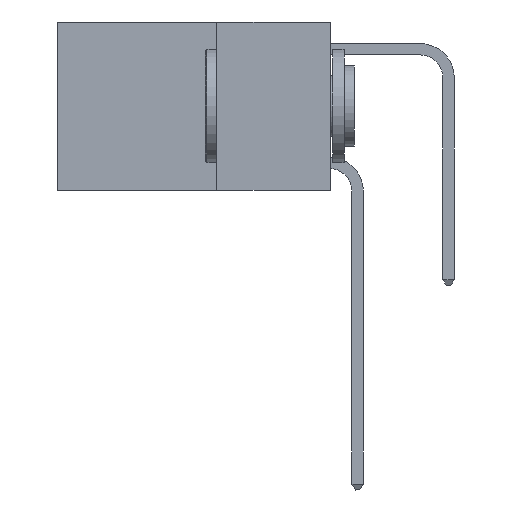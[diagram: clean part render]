
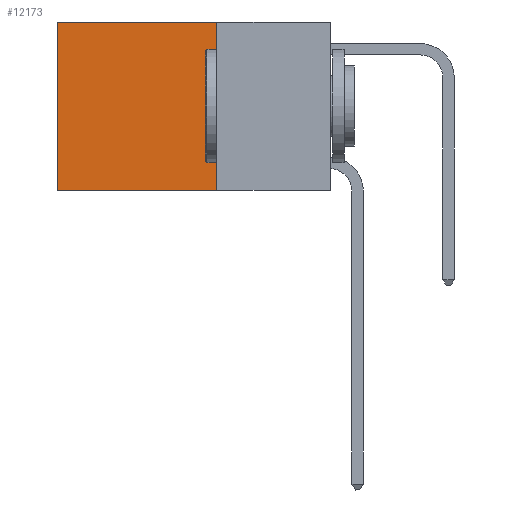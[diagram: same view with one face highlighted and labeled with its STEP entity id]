
A CAD part, left-side view. The second image highlights one B-rep face of the part: STEP entity #12173.
In plain terms, the highlighted planar face has unit normal (-1, 0, 0).
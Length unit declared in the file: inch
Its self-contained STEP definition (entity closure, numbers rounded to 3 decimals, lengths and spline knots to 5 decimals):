
#615 = VERTEX_POINT ( 'NONE', #9736 ) ;
#970 = EDGE_CURVE ( 'NONE', #3640, #1485, #16937, .T. ) ;
#1111 = DIRECTION ( 'NONE',  ( 0., 0., -1. ) ) ;
#1485 = VERTEX_POINT ( 'NONE', #8193 ) ;
#2724 = LINE ( 'NONE', #4094, #6900 ) ;
#2854 = DIRECTION ( 'NONE',  ( 0., 1., 0. ) ) ;
#3399 = EDGE_CURVE ( 'NONE', #615, #3640, #2724, .T. ) ;
#3640 = VERTEX_POINT ( 'NONE', #19001 ) ;
#4094 = CARTESIAN_POINT ( 'NONE',  ( 0.2625, 0.25, 0. ) ) ;
#4179 = CARTESIAN_POINT ( 'NONE',  ( 0.2625, 0.6, 0. ) ) ;
#4950 = AXIS2_PLACEMENT_3D ( 'NONE', #6698, #14297, #1111 ) ;
#5082 = ORIENTED_EDGE ( 'NONE', *, *, #23337, .T. ) ;
#5183 = ORIENTED_EDGE ( 'NONE', *, *, #970, .F. ) ;
#5208 = PLANE ( 'NONE',  #4950 ) ;
#5256 = CARTESIAN_POINT ( 'NONE',  ( 0.2625, 0.6, 0. ) ) ;
#6097 = VECTOR ( 'NONE', #2854, 39.37008 ) ;
#6468 = LINE ( 'NONE', #20037, #6097 ) ;
#6698 = CARTESIAN_POINT ( 'NONE',  ( 0.2625, 0.25, 0. ) ) ;
#6900 = VECTOR ( 'NONE', #8443, 39.37008 ) ;
#7489 = DIRECTION ( 'NONE',  ( 0., 1., 0. ) ) ;
#8166 = VECTOR ( 'NONE', #11771, 39.37008 ) ;
#8193 = CARTESIAN_POINT ( 'NONE',  ( 0.2625, 0.6, -0.37 ) ) ;
#8443 = DIRECTION ( 'NONE',  ( 0., 0., -1. ) ) ;
#9736 = CARTESIAN_POINT ( 'NONE',  ( 0.2625, 0.25, 0. ) ) ;
#10305 = VECTOR ( 'NONE', #7489, 39.37008 ) ;
#10434 = FACE_OUTER_BOUND ( 'NONE', #13181, .T. ) ;
#11771 = DIRECTION ( 'NONE',  ( 0., 0., -1. ) ) ;
#12173 = ADVANCED_FACE ( 'NONE', ( #10434 ), #5208, .F. ) ;
#13138 = LINE ( 'NONE', #4179, #8166 ) ;
#13181 = EDGE_LOOP ( 'NONE', ( #5082, #5183, #24292, #24544 ) ) ;
#14297 = DIRECTION ( 'NONE',  ( 1., 0., 0. ) ) ;
#16937 = LINE ( 'NONE', #17169, #10305 ) ;
#17169 = CARTESIAN_POINT ( 'NONE',  ( 0.2625, 0.25, -0.37 ) ) ;
#19001 = CARTESIAN_POINT ( 'NONE',  ( 0.2625, 0.25, -0.37 ) ) ;
#20037 = CARTESIAN_POINT ( 'NONE',  ( 0.2625, 0.25, 0. ) ) ;
#21068 = EDGE_CURVE ( 'NONE', #615, #24075, #6468, .T. ) ;
#23337 = EDGE_CURVE ( 'NONE', #24075, #1485, #13138, .T. ) ;
#24075 = VERTEX_POINT ( 'NONE', #5256 ) ;
#24292 = ORIENTED_EDGE ( 'NONE', *, *, #3399, .F. ) ;
#24544 = ORIENTED_EDGE ( 'NONE', *, *, #21068, .T. ) ;
